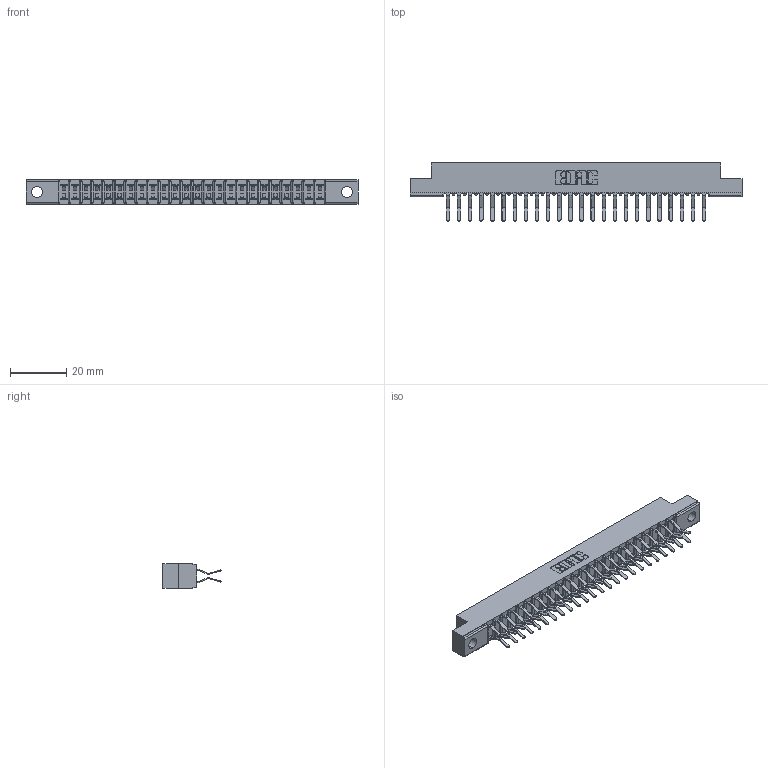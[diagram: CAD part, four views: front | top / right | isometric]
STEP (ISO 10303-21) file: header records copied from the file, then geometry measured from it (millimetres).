
FILE_DESCRIPTION (( 'STEP AP203' ), '1' );
FILE_NAME ('357-048-560-204.STEP', '2019-09-18T10:18:30', ( '' ), ( '' ), 'SwSTEP 2.0', 'SolidWorks 2016', '' );
FILE_SCHEMA (( 'CONFIG_CONTROL_DESIGN' ));
Length unit declared in the file: inch
Products named in the file (3): 307-290-001_560; 307 Part_.156 Dia Mounting Holes; 357-048-560-204
Assembly tree (49 placements, depth 2):
  357-048-560-204
    307 Part_.156 Dia Mounting Holes
    307-290-001_560  x48
Bounding box: 118.11 x 20.73 x 8.71 mm (x, y, z)
Volume: 7679.3 mm3; surface area: 13919.7 mm2
Topology: 49 solids, 49 shells, 2557 faces, 7175 edges, 4650 vertices
Faces by surface type: plane 1668, cylinder 839, sphere 50
Entity records: 24084 total; most frequent: CARTESIAN_POINT 3950, ORIENTED_EDGE 3910, DIRECTION 3869, EDGE_CURVE 1955, VECTOR 1499, LINE 1499, VERTEX_POINT 1266, AXIS2_PLACEMENT_3D 1185
